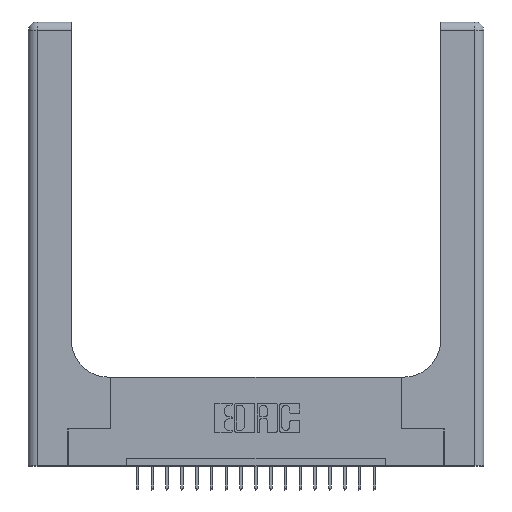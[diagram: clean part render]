
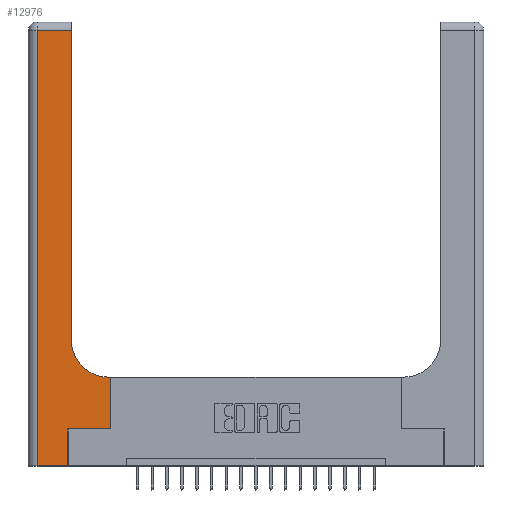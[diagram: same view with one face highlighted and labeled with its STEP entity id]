
A CAD part, top view. The second image highlights one B-rep face of the part: STEP entity #12976.
In plain terms, the highlighted planar face has unit normal (0, 0, 1).
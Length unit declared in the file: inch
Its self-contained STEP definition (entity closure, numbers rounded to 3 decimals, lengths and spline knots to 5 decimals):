
#222 = EDGE_CURVE ( 'NONE', #11200, #20630, #11071, .T. ) ;
#340 = DIRECTION ( 'NONE',  ( 0., 1., 0. ) ) ;
#379 = FACE_OUTER_BOUND ( 'NONE', #16367, .T. ) ;
#411 = CARTESIAN_POINT ( 'NONE',  ( 0.269, 0., 0.37 ) ) ;
#984 = VERTEX_POINT ( 'NONE', #5470 ) ;
#1085 = PLANE ( 'NONE',  #17977 ) ;
#1562 = DIRECTION ( 'NONE',  ( -1., 0., 0. ) ) ;
#2198 = CARTESIAN_POINT ( 'NONE',  ( 0.269, 0., 0.37 ) ) ;
#2252 = DIRECTION ( 'NONE',  ( -1., 0., 0. ) ) ;
#2401 = ORIENTED_EDGE ( 'NONE', *, *, #11975, .T. ) ;
#2697 = CARTESIAN_POINT ( 'NONE',  ( 0.06, 0., 0.37 ) ) ;
#2899 = CARTESIAN_POINT ( 'NONE',  ( 0.2915, 0.6, 0.37 ) ) ;
#2956 = DIRECTION ( 'NONE',  ( 1., 0., 0. ) ) ;
#3058 = AXIS2_PLACEMENT_3D ( 'NONE', #20894, #5891, #17458 ) ;
#3203 = EDGE_CURVE ( 'NONE', #8826, #5439, #7519, .T. ) ;
#3330 = VECTOR ( 'NONE', #4099, 39.37008 ) ;
#3744 = ORIENTED_EDGE ( 'NONE', *, *, #7140, .T. ) ;
#3809 = LINE ( 'NONE', #12215, #20838 ) ;
#4099 = DIRECTION ( 'NONE',  ( 0., 1., 0. ) ) ;
#4554 = CARTESIAN_POINT ( 'NONE',  ( 0.269, 0.25, 0.37 ) ) ;
#4591 = CARTESIAN_POINT ( 'NONE',  ( 0., 3., 0.37 ) ) ;
#5035 = CARTESIAN_POINT ( 'NONE',  ( 0.2915, 2.94, 0.37 ) ) ;
#5229 = CARTESIAN_POINT ( 'NONE',  ( 0.06, 2.94, 0.37 ) ) ;
#5439 = VERTEX_POINT ( 'NONE', #2198 ) ;
#5470 = CARTESIAN_POINT ( 'NONE',  ( 0.269, 0.25, 0.37 ) ) ;
#5741 = LINE ( 'NONE', #20850, #20729 ) ;
#5776 = LINE ( 'NONE', #2899, #8140 ) ;
#5799 = LINE ( 'NONE', #15709, #18772 ) ;
#5891 = DIRECTION ( 'NONE',  ( 0., 0., -1. ) ) ;
#6296 = EDGE_CURVE ( 'NONE', #21056, #14470, #5799, .T. ) ;
#6550 = CARTESIAN_POINT ( 'NONE',  ( 0.5415, 0.6, 0.37 ) ) ;
#6811 = ORIENTED_EDGE ( 'NONE', *, *, #3203, .T. ) ;
#7140 = EDGE_CURVE ( 'NONE', #20630, #11900, #5776, .T. ) ;
#7519 = LINE ( 'NONE', #13702, #11896 ) ;
#8140 = VECTOR ( 'NONE', #2252, 39.37008 ) ;
#8711 = ORIENTED_EDGE ( 'NONE', *, *, #10103, .T. ) ;
#8753 = DIRECTION ( 'NONE',  ( 1., 0., 0. ) ) ;
#8798 = CIRCLE ( 'NONE', #3058, 0.25 ) ;
#8826 = VERTEX_POINT ( 'NONE', #2697 ) ;
#9261 = CARTESIAN_POINT ( 'NONE',  ( 0.5585, 0.6, 0.37 ) ) ;
#9331 = VECTOR ( 'NONE', #2956, 39.37008 ) ;
#9784 = ORIENTED_EDGE ( 'NONE', *, *, #16462, .T. ) ;
#9847 = LINE ( 'NONE', #4554, #9331 ) ;
#10103 = EDGE_CURVE ( 'NONE', #984, #11200, #9847, .T. ) ;
#10536 = CARTESIAN_POINT ( 'NONE',  ( 0.5585, 0.25, 0.37 ) ) ;
#10835 = ORIENTED_EDGE ( 'NONE', *, *, #20580, .T. ) ;
#10886 = CARTESIAN_POINT ( 'NONE',  ( 0.5585, 0.25, 0.37 ) ) ;
#11071 = LINE ( 'NONE', #10536, #3330 ) ;
#11132 = ORIENTED_EDGE ( 'NONE', *, *, #17155, .T. ) ;
#11200 = VERTEX_POINT ( 'NONE', #10886 ) ;
#11896 = VECTOR ( 'NONE', #8753, 39.37008 ) ;
#11900 = VERTEX_POINT ( 'NONE', #6550 ) ;
#11975 = EDGE_CURVE ( 'NONE', #13223, #8826, #3809, .T. ) ;
#12215 = CARTESIAN_POINT ( 'NONE',  ( 0.06, 3., 0.37 ) ) ;
#12976 = ADVANCED_FACE ( 'NONE', ( #379 ), #1085, .F. ) ;
#13223 = VERTEX_POINT ( 'NONE', #5229 ) ;
#13312 = ORIENTED_EDGE ( 'NONE', *, *, #222, .T. ) ;
#13702 = CARTESIAN_POINT ( 'NONE',  ( 0., 0., 0.37 ) ) ;
#13957 = LINE ( 'NONE', #411, #15267 ) ;
#14426 = DIRECTION ( 'NONE',  ( 0., 0., -1. ) ) ;
#14470 = VERTEX_POINT ( 'NONE', #5035 ) ;
#15138 = ORIENTED_EDGE ( 'NONE', *, *, #6296, .T. ) ;
#15267 = VECTOR ( 'NONE', #340, 39.37008 ) ;
#15709 = CARTESIAN_POINT ( 'NONE',  ( 0.2915, 3., 0.37 ) ) ;
#16367 = EDGE_LOOP ( 'NONE', ( #15138, #10835, #2401, #6811, #9784, #8711, #13312, #3744, #11132 ) ) ;
#16462 = EDGE_CURVE ( 'NONE', #5439, #984, #13957, .T. ) ;
#17155 = EDGE_CURVE ( 'NONE', #11900, #21056, #8798, .T. ) ;
#17452 = CARTESIAN_POINT ( 'NONE',  ( 0.2915, 0.85, 0.37 ) ) ;
#17458 = DIRECTION ( 'NONE',  ( 1., 0., 0. ) ) ;
#17977 = AXIS2_PLACEMENT_3D ( 'NONE', #4591, #14426, #19398 ) ;
#18772 = VECTOR ( 'NONE', #18829, 39.37008 ) ;
#18829 = DIRECTION ( 'NONE',  ( 0., 1., 0. ) ) ;
#19398 = DIRECTION ( 'NONE',  ( -1., 0., 0. ) ) ;
#20526 = DIRECTION ( 'NONE',  ( 0., -1., 0. ) ) ;
#20580 = EDGE_CURVE ( 'NONE', #14470, #13223, #5741, .T. ) ;
#20630 = VERTEX_POINT ( 'NONE', #9261 ) ;
#20729 = VECTOR ( 'NONE', #1562, 39.37008 ) ;
#20838 = VECTOR ( 'NONE', #20526, 39.37008 ) ;
#20850 = CARTESIAN_POINT ( 'NONE',  ( 0., 2.94, 0.37 ) ) ;
#20894 = CARTESIAN_POINT ( 'NONE',  ( 0.5415, 0.85, 0.37 ) ) ;
#21056 = VERTEX_POINT ( 'NONE', #17452 ) ;
